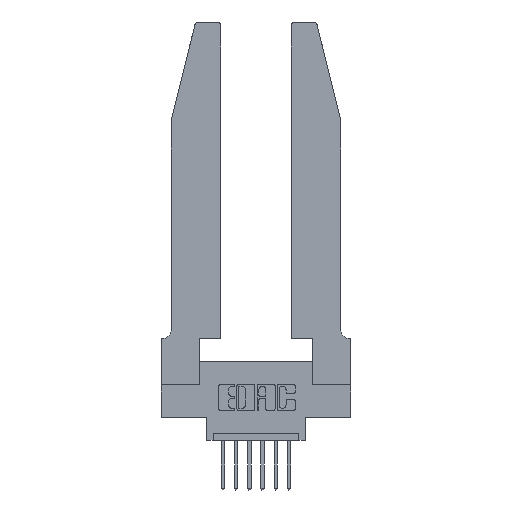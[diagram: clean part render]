
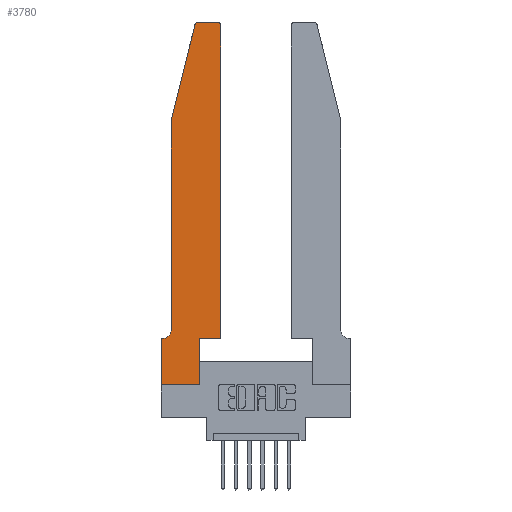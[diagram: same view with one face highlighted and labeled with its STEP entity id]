
A CAD part, top view. The second image highlights one B-rep face of the part: STEP entity #3780.
In plain terms, the highlighted planar face has unit normal (0, 0, 1).
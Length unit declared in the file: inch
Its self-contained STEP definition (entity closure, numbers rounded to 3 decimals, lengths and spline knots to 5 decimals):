
#158 = CARTESIAN_POINT ( 'NONE',  ( 0.4505, 0.35, 0.37 ) ) ;
#260 = AXIS2_PLACEMENT_3D ( 'NONE', #6890, #7936, #11152 ) ;
#343 = CARTESIAN_POINT ( 'NONE',  ( 0.2865, 0., 0.37 ) ) ;
#566 = VECTOR ( 'NONE', #1986, 39.37008 ) ;
#590 = DIRECTION ( 'NONE',  ( 0., 0., -1. ) ) ;
#633 = VECTOR ( 'NONE', #13220, 39.37008 ) ;
#704 = CARTESIAN_POINT ( 'NONE',  ( 0.0055, 0.35, 0.37 ) ) ;
#1046 = EDGE_CURVE ( 'NONE', #4815, #7972, #3048, .T. ) ;
#1061 = EDGE_CURVE ( 'NONE', #10316, #13169, #4593, .T. ) ;
#1265 = CARTESIAN_POINT ( 'NONE',  ( 0.284, 2.75, 0.37 ) ) ;
#1289 = DIRECTION ( 'NONE',  ( 0., 0., 1. ) ) ;
#1308 = DIRECTION ( 'NONE',  ( 0., -1., 0. ) ) ;
#1344 = VECTOR ( 'NONE', #13392, 39.37008 ) ;
#1383 = CARTESIAN_POINT ( 'NONE',  ( 0., 0.35, 0.37 ) ) ;
#1645 = VERTEX_POINT ( 'NONE', #4762 ) ;
#1778 = EDGE_CURVE ( 'NONE', #13706, #4815, #2478, .T. ) ;
#1986 = DIRECTION ( 'NONE',  ( 0., 1., 0. ) ) ;
#2062 = EDGE_CURVE ( 'NONE', #12902, #4198, #2656, .T. ) ;
#2478 = LINE ( 'NONE', #3196, #13546 ) ;
#2490 = CARTESIAN_POINT ( 'NONE',  ( 0.0755, 0.42, 0.37 ) ) ;
#2513 = VECTOR ( 'NONE', #6949, 39.37008 ) ;
#2516 = CARTESIAN_POINT ( 'NONE',  ( 0.284, 2.72, 0.37 ) ) ;
#2656 = CIRCLE ( 'NONE', #6971, 0.03 ) ;
#2733 = ORIENTED_EDGE ( 'NONE', *, *, #1778, .T. ) ;
#3048 = LINE ( 'NONE', #12932, #11516 ) ;
#3158 = LINE ( 'NONE', #6357, #566 ) ;
#3190 = VERTEX_POINT ( 'NONE', #4107 ) ;
#3196 = CARTESIAN_POINT ( 'NONE',  ( 0., 0., 0.37 ) ) ;
#3494 = CARTESIAN_POINT ( 'NONE',  ( 0., 0., 0.37 ) ) ;
#3780 = ADVANCED_FACE ( 'NONE', ( #9339 ), #12300, .T. ) ;
#3961 = CARTESIAN_POINT ( 'NONE',  ( 0., 0., 0.37 ) ) ;
#4107 = CARTESIAN_POINT ( 'NONE',  ( 0.0755, 2., 0.37 ) ) ;
#4119 = ORIENTED_EDGE ( 'NONE', *, *, #13962, .T. ) ;
#4198 = VERTEX_POINT ( 'NONE', #7149 ) ;
#4573 = CARTESIAN_POINT ( 'NONE',  ( 0.0755, 0.35, 0.37 ) ) ;
#4593 = CIRCLE ( 'NONE', #9285, 0.07 ) ;
#4747 = DIRECTION ( 'NONE',  ( 0., 0., 1. ) ) ;
#4762 = CARTESIAN_POINT ( 'NONE',  ( 0.4505, 2.72, 0.37 ) ) ;
#4815 = VERTEX_POINT ( 'NONE', #343 ) ;
#4926 = LINE ( 'NONE', #12552, #9918 ) ;
#5332 = DIRECTION ( 'NONE',  ( 1., 0., 0. ) ) ;
#5853 = DIRECTION ( 'NONE',  ( 1., 0., 0. ) ) ;
#5940 = ORIENTED_EDGE ( 'NONE', *, *, #8032, .T. ) ;
#6183 = LINE ( 'NONE', #3494, #9467 ) ;
#6287 = VERTEX_POINT ( 'NONE', #1383 ) ;
#6357 = CARTESIAN_POINT ( 'NONE',  ( 0.4505, 0.35, 0.37 ) ) ;
#6462 = EDGE_CURVE ( 'NONE', #13169, #6287, #7870, .T. ) ;
#6805 = CARTESIAN_POINT ( 'NONE',  ( 0.2605, 2.75, 0.37 ) ) ;
#6847 = CARTESIAN_POINT ( 'NONE',  ( 0.4205, 2.72, 0.37 ) ) ;
#6881 = ORIENTED_EDGE ( 'NONE', *, *, #2062, .T. ) ;
#6890 = CARTESIAN_POINT ( 'NONE',  ( 0., 0.35, 0.37 ) ) ;
#6949 = DIRECTION ( 'NONE',  ( -1., 0., 0. ) ) ;
#6971 = AXIS2_PLACEMENT_3D ( 'NONE', #2516, #4747, #5853 ) ;
#7087 = ORIENTED_EDGE ( 'NONE', *, *, #1061, .T. ) ;
#7149 = CARTESIAN_POINT ( 'NONE',  ( 0.25487, 2.72718, 0.37 ) ) ;
#7376 = EDGE_CURVE ( 'NONE', #12286, #12902, #12037, .T. ) ;
#7430 = AXIS2_PLACEMENT_3D ( 'NONE', #6847, #1289, #11405 ) ;
#7870 = LINE ( 'NONE', #4573, #633 ) ;
#7936 = DIRECTION ( 'NONE',  ( 0., 0., 1. ) ) ;
#7960 = CARTESIAN_POINT ( 'NONE',  ( 0.0755, 2., 0.37 ) ) ;
#7972 = VERTEX_POINT ( 'NONE', #13341 ) ;
#8032 = EDGE_CURVE ( 'NONE', #7972, #10330, #11843, .T. ) ;
#8050 = ORIENTED_EDGE ( 'NONE', *, *, #7376, .T. ) ;
#9049 = VECTOR ( 'NONE', #10308, 39.37008 ) ;
#9081 = ORIENTED_EDGE ( 'NONE', *, *, #1046, .T. ) ;
#9139 = DIRECTION ( 'NONE',  ( -0.239, -0.971, 0. ) ) ;
#9285 = AXIS2_PLACEMENT_3D ( 'NONE', #10601, #590, #12642 ) ;
#9319 = ORIENTED_EDGE ( 'NONE', *, *, #11376, .T. ) ;
#9339 = FACE_OUTER_BOUND ( 'NONE', #11032, .T. ) ;
#9467 = VECTOR ( 'NONE', #1308, 39.37008 ) ;
#9918 = VECTOR ( 'NONE', #9139, 39.37008 ) ;
#10308 = DIRECTION ( 'NONE',  ( 1., 0., 0. ) ) ;
#10316 = VERTEX_POINT ( 'NONE', #2490 ) ;
#10330 = VERTEX_POINT ( 'NONE', #13652 ) ;
#10514 = LINE ( 'NONE', #7960, #1344 ) ;
#10601 = CARTESIAN_POINT ( 'NONE',  ( 0.0055, 0.42, 0.37 ) ) ;
#10753 = EDGE_CURVE ( 'NONE', #3190, #10316, #10514, .T. ) ;
#10788 = EDGE_CURVE ( 'NONE', #6287, #13706, #6183, .T. ) ;
#11032 = EDGE_LOOP ( 'NONE', ( #8050, #6881, #12990, #12450, #7087, #11350, #13621, #2733, #9081, #5940, #4119, #9319 ) ) ;
#11152 = DIRECTION ( 'NONE',  ( 1., 0., 0. ) ) ;
#11350 = ORIENTED_EDGE ( 'NONE', *, *, #6462, .T. ) ;
#11376 = EDGE_CURVE ( 'NONE', #1645, #12286, #12589, .T. ) ;
#11405 = DIRECTION ( 'NONE',  ( 1., 0., 0. ) ) ;
#11516 = VECTOR ( 'NONE', #11716, 39.37008 ) ;
#11716 = DIRECTION ( 'NONE',  ( 0., 1., 0. ) ) ;
#11843 = LINE ( 'NONE', #158, #9049 ) ;
#12010 = CARTESIAN_POINT ( 'NONE',  ( 0.4205, 2.75, 0.37 ) ) ;
#12037 = LINE ( 'NONE', #6805, #2513 ) ;
#12286 = VERTEX_POINT ( 'NONE', #12010 ) ;
#12300 = PLANE ( 'NONE',  #260 ) ;
#12450 = ORIENTED_EDGE ( 'NONE', *, *, #10753, .T. ) ;
#12552 = CARTESIAN_POINT ( 'NONE',  ( 0.0755, 2., 0.37 ) ) ;
#12589 = CIRCLE ( 'NONE', #7430, 0.03 ) ;
#12642 = DIRECTION ( 'NONE',  ( -1., 0., 0. ) ) ;
#12902 = VERTEX_POINT ( 'NONE', #1265 ) ;
#12932 = CARTESIAN_POINT ( 'NONE',  ( 0.2865, 0.35, 0.37 ) ) ;
#12970 = EDGE_CURVE ( 'NONE', #4198, #3190, #4926, .T. ) ;
#12990 = ORIENTED_EDGE ( 'NONE', *, *, #12970, .T. ) ;
#13169 = VERTEX_POINT ( 'NONE', #704 ) ;
#13220 = DIRECTION ( 'NONE',  ( -1., 0., 0. ) ) ;
#13341 = CARTESIAN_POINT ( 'NONE',  ( 0.2865, 0.35, 0.37 ) ) ;
#13392 = DIRECTION ( 'NONE',  ( 0., -1., 0. ) ) ;
#13546 = VECTOR ( 'NONE', #5332, 39.37008 ) ;
#13621 = ORIENTED_EDGE ( 'NONE', *, *, #10788, .T. ) ;
#13652 = CARTESIAN_POINT ( 'NONE',  ( 0.4505, 0.35, 0.37 ) ) ;
#13706 = VERTEX_POINT ( 'NONE', #3961 ) ;
#13962 = EDGE_CURVE ( 'NONE', #10330, #1645, #3158, .T. ) ;
